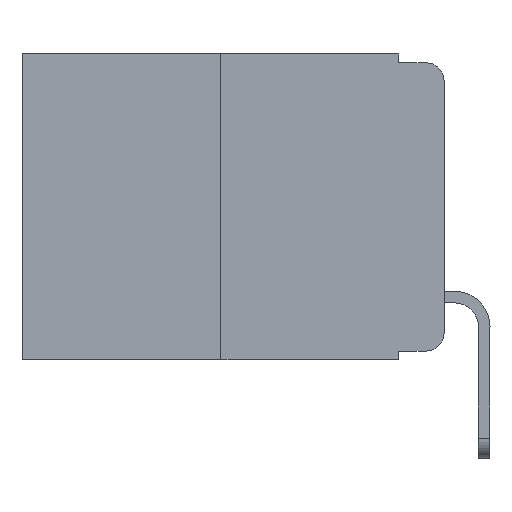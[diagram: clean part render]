
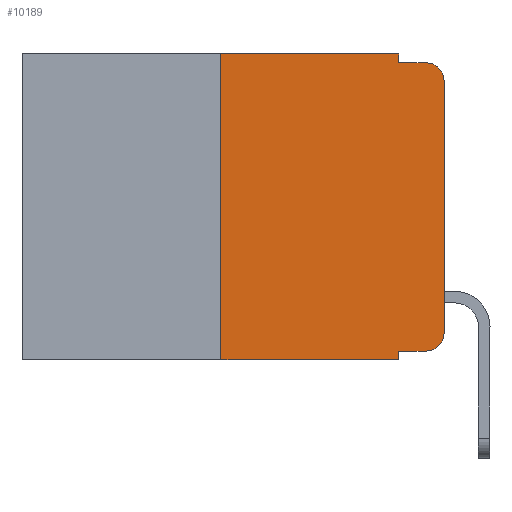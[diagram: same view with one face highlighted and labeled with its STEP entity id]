
A CAD part, left-side view. The second image highlights one B-rep face of the part: STEP entity #10189.
In plain terms, the highlighted planar face has unit normal (-1, 0, 0).
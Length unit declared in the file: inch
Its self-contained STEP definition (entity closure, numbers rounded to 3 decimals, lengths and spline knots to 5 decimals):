
#194 = CARTESIAN_POINT ( 'NONE',  ( 0., 0.02, -0.333 ) ) ;
#296 = EDGE_CURVE ( 'NONE', #18817, #20803, #14029, .T. ) ;
#342 = CARTESIAN_POINT ( 'NONE',  ( 0., 0.02, -0.313 ) ) ;
#1751 = VECTOR ( 'NONE', #2643, 39.37008 ) ;
#2070 = CARTESIAN_POINT ( 'NONE',  ( 0., 0.051, 0. ) ) ;
#2198 = DIRECTION ( 'NONE',  ( -1., 0., 0. ) ) ;
#2208 = VERTEX_POINT ( 'NONE', #11206 ) ;
#2468 = CIRCLE ( 'NONE', #21646, 0.02 ) ;
#2643 = DIRECTION ( 'NONE',  ( 0., 0., 1. ) ) ;
#2688 = EDGE_CURVE ( 'NONE', #8807, #2208, #13352, .T. ) ;
#3957 = ORIENTED_EDGE ( 'NONE', *, *, #296, .F. ) ;
#4429 = PLANE ( 'NONE',  #7050 ) ;
#4879 = DIRECTION ( 'NONE',  ( 0., -1., 0. ) ) ;
#5001 = VERTEX_POINT ( 'NONE', #6647 ) ;
#5427 = CARTESIAN_POINT ( 'NONE',  ( 0., 0.02, -0.03 ) ) ;
#5499 = CIRCLE ( 'NONE', #19466, 0.02 ) ;
#5617 = LINE ( 'NONE', #16954, #11879 ) ;
#6220 = ORIENTED_EDGE ( 'NONE', *, *, #2688, .T. ) ;
#6487 = DIRECTION ( 'NONE',  ( 0., 0., -1. ) ) ;
#6647 = CARTESIAN_POINT ( 'NONE',  ( 0., 0.051, -0.333 ) ) ;
#6775 = VECTOR ( 'NONE', #4879, 39.37008 ) ;
#7050 = AXIS2_PLACEMENT_3D ( 'NONE', #11655, #9953, #13417 ) ;
#7363 = DIRECTION ( 'NONE',  ( 0., 0., -1. ) ) ;
#7409 = VERTEX_POINT ( 'NONE', #16158 ) ;
#7559 = EDGE_CURVE ( 'NONE', #5001, #21452, #21895, .T. ) ;
#7996 = LINE ( 'NONE', #11892, #13754 ) ;
#8010 = CARTESIAN_POINT ( 'NONE',  ( 0., 0., -0.313 ) ) ;
#8318 = CARTESIAN_POINT ( 'NONE',  ( 0., 0.051, -0.333 ) ) ;
#8744 = VECTOR ( 'NONE', #13883, 39.37008 ) ;
#8807 = VERTEX_POINT ( 'NONE', #14231 ) ;
#9412 = EDGE_CURVE ( 'NONE', #5001, #2208, #21468, .T. ) ;
#9772 = EDGE_LOOP ( 'NONE', ( #19504, #10106, #22617, #15340, #3957, #11084, #6220, #15833, #14069, #16107 ) ) ;
#9953 = DIRECTION ( 'NONE',  ( 1., 0., 0. ) ) ;
#10106 = ORIENTED_EDGE ( 'NONE', *, *, #17914, .T. ) ;
#10189 = ADVANCED_FACE ( 'NONE', ( #20095 ), #4429, .F. ) ;
#10513 = VERTEX_POINT ( 'NONE', #17381 ) ;
#10841 = VERTEX_POINT ( 'NONE', #8010 ) ;
#11084 = ORIENTED_EDGE ( 'NONE', *, *, #16344, .F. ) ;
#11206 = CARTESIAN_POINT ( 'NONE',  ( 0., 0.051, -0.343 ) ) ;
#11655 = CARTESIAN_POINT ( 'NONE',  ( 0., 0.473, 0. ) ) ;
#11784 = DIRECTION ( 'NONE',  ( 0., -1., 0. ) ) ;
#11815 = CARTESIAN_POINT ( 'NONE',  ( 0., 0.473, -0.343 ) ) ;
#11879 = VECTOR ( 'NONE', #6487, 39.37008 ) ;
#11892 = CARTESIAN_POINT ( 'NONE',  ( 0., 0., 0. ) ) ;
#12077 = CARTESIAN_POINT ( 'NONE',  ( 0., 0.051, -0.01 ) ) ;
#12142 = CARTESIAN_POINT ( 'NONE',  ( 0., 0.051, -0.01 ) ) ;
#12649 = CARTESIAN_POINT ( 'NONE',  ( 0., 0.051, 0. ) ) ;
#12794 = EDGE_CURVE ( 'NONE', #15416, #10513, #21615, .T. ) ;
#12971 = CARTESIAN_POINT ( 'NONE',  ( 0., 0.25, 0. ) ) ;
#13352 = LINE ( 'NONE', #11815, #6775 ) ;
#13417 = DIRECTION ( 'NONE',  ( 0., 0., -1. ) ) ;
#13754 = VECTOR ( 'NONE', #18631, 39.37008 ) ;
#13883 = DIRECTION ( 'NONE',  ( 0., -1., 0. ) ) ;
#14029 = LINE ( 'NONE', #19885, #20063 ) ;
#14069 = ORIENTED_EDGE ( 'NONE', *, *, #7559, .T. ) ;
#14231 = CARTESIAN_POINT ( 'NONE',  ( 0., 0.25, -0.343 ) ) ;
#14386 = DIRECTION ( 'NONE',  ( -1., 0., 0. ) ) ;
#14411 = DIRECTION ( 'NONE',  ( 0., 0., -1. ) ) ;
#15071 = VECTOR ( 'NONE', #11784, 39.37008 ) ;
#15340 = ORIENTED_EDGE ( 'NONE', *, *, #21052, .F. ) ;
#15416 = VERTEX_POINT ( 'NONE', #12077 ) ;
#15833 = ORIENTED_EDGE ( 'NONE', *, *, #9412, .F. ) ;
#16107 = ORIENTED_EDGE ( 'NONE', *, *, #19077, .T. ) ;
#16158 = CARTESIAN_POINT ( 'NONE',  ( 0., 0., -0.03 ) ) ;
#16344 = EDGE_CURVE ( 'NONE', #8807, #18817, #16764, .T. ) ;
#16764 = LINE ( 'NONE', #12971, #1751 ) ;
#16954 = CARTESIAN_POINT ( 'NONE',  ( 0., 0.051, 0. ) ) ;
#17381 = CARTESIAN_POINT ( 'NONE',  ( 0., 0.02, -0.01 ) ) ;
#17909 = DIRECTION ( 'NONE',  ( 0., 0., -1. ) ) ;
#17914 = EDGE_CURVE ( 'NONE', #7409, #10513, #5499, .T. ) ;
#18203 = VECTOR ( 'NONE', #7363, 39.37008 ) ;
#18631 = DIRECTION ( 'NONE',  ( 0., 0., 1. ) ) ;
#18817 = VERTEX_POINT ( 'NONE', #20808 ) ;
#19077 = EDGE_CURVE ( 'NONE', #21452, #10841, #2468, .T. ) ;
#19466 = AXIS2_PLACEMENT_3D ( 'NONE', #5427, #2198, #14411 ) ;
#19504 = ORIENTED_EDGE ( 'NONE', *, *, #21207, .T. ) ;
#19885 = CARTESIAN_POINT ( 'NONE',  ( 0., 0.473, 0. ) ) ;
#20063 = VECTOR ( 'NONE', #21303, 39.37008 ) ;
#20095 = FACE_OUTER_BOUND ( 'NONE', #9772, .T. ) ;
#20803 = VERTEX_POINT ( 'NONE', #12649 ) ;
#20808 = CARTESIAN_POINT ( 'NONE',  ( 0., 0.25, 0. ) ) ;
#21052 = EDGE_CURVE ( 'NONE', #20803, #15416, #5617, .T. ) ;
#21207 = EDGE_CURVE ( 'NONE', #10841, #7409, #7996, .T. ) ;
#21303 = DIRECTION ( 'NONE',  ( 0., -1., 0. ) ) ;
#21452 = VERTEX_POINT ( 'NONE', #194 ) ;
#21468 = LINE ( 'NONE', #2070, #18203 ) ;
#21615 = LINE ( 'NONE', #12142, #8744 ) ;
#21646 = AXIS2_PLACEMENT_3D ( 'NONE', #342, #14386, #17909 ) ;
#21895 = LINE ( 'NONE', #8318, #15071 ) ;
#22617 = ORIENTED_EDGE ( 'NONE', *, *, #12794, .F. ) ;
